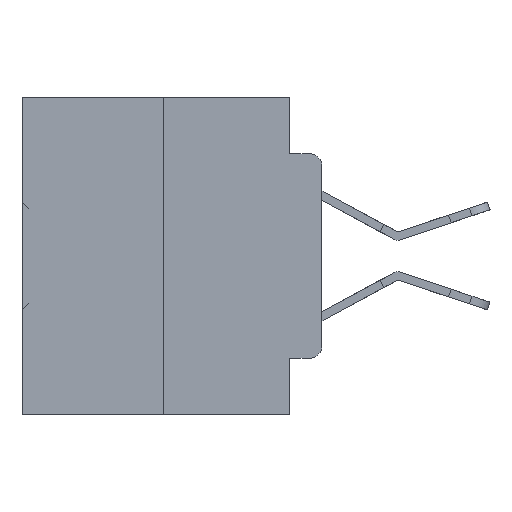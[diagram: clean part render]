
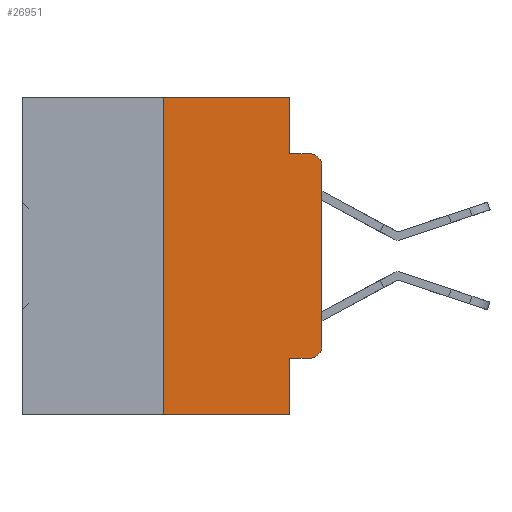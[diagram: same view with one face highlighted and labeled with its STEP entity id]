
A CAD part, left-side view. The second image highlights one B-rep face of the part: STEP entity #26951.
In plain terms, the highlighted planar face has unit normal (-1, 0, 0).
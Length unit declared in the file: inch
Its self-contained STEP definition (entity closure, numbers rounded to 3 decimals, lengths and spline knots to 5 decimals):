
#3 = EDGE_CURVE ( 'NONE', #21176, #24226, #10777, .T. ) ;
#64 = CARTESIAN_POINT ( 'NONE',  ( 0., 0.473, 0. ) ) ;
#279 = ORIENTED_EDGE ( 'NONE', *, *, #30904, .T. ) ;
#1422 = CARTESIAN_POINT ( 'NONE',  ( 0., 0.051, -0.0885 ) ) ;
#1730 = DIRECTION ( 'NONE',  ( 0., 0., 1. ) ) ;
#2903 = CIRCLE ( 'NONE', #6077, 0.02 ) ;
#4366 = CIRCLE ( 'NONE', #36384, 0.02 ) ;
#4468 = VECTOR ( 'NONE', #33080, 39.37008 ) ;
#5482 = LINE ( 'NONE', #11292, #4468 ) ;
#5577 = DIRECTION ( 'NONE',  ( 0., -1., 0. ) ) ;
#5899 = ORIENTED_EDGE ( 'NONE', *, *, #18908, .T. ) ;
#6077 = AXIS2_PLACEMENT_3D ( 'NONE', #33040, #14401, #36176 ) ;
#6322 = DIRECTION ( 'NONE',  ( -1., 0., 0. ) ) ;
#6934 = CARTESIAN_POINT ( 'NONE',  ( 0., 0.051, -0.4115 ) ) ;
#7149 = VECTOR ( 'NONE', #20381, 39.37008 ) ;
#7577 = CARTESIAN_POINT ( 'NONE',  ( 0., 0.051, 0. ) ) ;
#9055 = CARTESIAN_POINT ( 'NONE',  ( 0., 0., -0.3915 ) ) ;
#9959 = VECTOR ( 'NONE', #37285, 39.37008 ) ;
#10777 = LINE ( 'NONE', #7577, #18119 ) ;
#10796 = LINE ( 'NONE', #33046, #35670 ) ;
#10848 = CARTESIAN_POINT ( 'NONE',  ( 0., 0.051, -0.4115 ) ) ;
#11292 = CARTESIAN_POINT ( 'NONE',  ( 0., 0.473, -0.5 ) ) ;
#11466 = EDGE_CURVE ( 'NONE', #22764, #39345, #26602, .T. ) ;
#12318 = ORIENTED_EDGE ( 'NONE', *, *, #29073, .F. ) ;
#12628 = VERTEX_POINT ( 'NONE', #28226 ) ;
#14401 = DIRECTION ( 'NONE',  ( -1., 0., 0. ) ) ;
#15330 = VERTEX_POINT ( 'NONE', #18679 ) ;
#15375 = VECTOR ( 'NONE', #35049, 39.37008 ) ;
#15908 = VECTOR ( 'NONE', #5577, 39.37008 ) ;
#16170 = VERTEX_POINT ( 'NONE', #19553 ) ;
#16199 = AXIS2_PLACEMENT_3D ( 'NONE', #64, #37818, #19176 ) ;
#16276 = ORIENTED_EDGE ( 'NONE', *, *, #22108, .F. ) ;
#16366 = LINE ( 'NONE', #6934, #15375 ) ;
#16507 = LINE ( 'NONE', #1422, #7149 ) ;
#16768 = LINE ( 'NONE', #27586, #19677 ) ;
#17166 = CARTESIAN_POINT ( 'NONE',  ( 0., 0., -0.1085 ) ) ;
#17254 = CARTESIAN_POINT ( 'NONE',  ( 0., 0.25, 0. ) ) ;
#18119 = VECTOR ( 'NONE', #25619, 39.37008 ) ;
#18137 = CARTESIAN_POINT ( 'NONE',  ( 0., 0.473, 0. ) ) ;
#18679 = CARTESIAN_POINT ( 'NONE',  ( 0., 0.02, -0.0885 ) ) ;
#18908 = EDGE_CURVE ( 'NONE', #22764, #24226, #5482, .T. ) ;
#19041 = PLANE ( 'NONE',  #16199 ) ;
#19176 = DIRECTION ( 'NONE',  ( 0., 0., -1. ) ) ;
#19553 = CARTESIAN_POINT ( 'NONE',  ( 0., 0.051, 0. ) ) ;
#19677 = VECTOR ( 'NONE', #30671, 39.37008 ) ;
#20381 = DIRECTION ( 'NONE',  ( 0., -1., 0. ) ) ;
#20750 = EDGE_CURVE ( 'NONE', #39345, #16170, #24199, .T. ) ;
#21176 = VERTEX_POINT ( 'NONE', #10848 ) ;
#21931 = ORIENTED_EDGE ( 'NONE', *, *, #25823, .T. ) ;
#22108 = EDGE_CURVE ( 'NONE', #16170, #28282, #16768, .T. ) ;
#22236 = EDGE_CURVE ( 'NONE', #36190, #15330, #4366, .T. ) ;
#22699 = CARTESIAN_POINT ( 'NONE',  ( 0., 0.051, -0.5 ) ) ;
#22764 = VERTEX_POINT ( 'NONE', #37313 ) ;
#23187 = EDGE_CURVE ( 'NONE', #36437, #36190, #10796, .T. ) ;
#24199 = LINE ( 'NONE', #18137, #15908 ) ;
#24226 = VERTEX_POINT ( 'NONE', #22699 ) ;
#25109 = CARTESIAN_POINT ( 'NONE',  ( 0., 0.02, -0.1085 ) ) ;
#25619 = DIRECTION ( 'NONE',  ( 0., 0., -1. ) ) ;
#25823 = EDGE_CURVE ( 'NONE', #12628, #36437, #2903, .T. ) ;
#26602 = LINE ( 'NONE', #34161, #9959 ) ;
#26951 = ADVANCED_FACE ( 'NONE', ( #36657 ), #19041, .F. ) ;
#27586 = CARTESIAN_POINT ( 'NONE',  ( 0., 0.051, 0. ) ) ;
#28226 = CARTESIAN_POINT ( 'NONE',  ( 0., 0.02, -0.4115 ) ) ;
#28244 = DIRECTION ( 'NONE',  ( 0., 0., -1. ) ) ;
#28282 = VERTEX_POINT ( 'NONE', #29022 ) ;
#28566 = ORIENTED_EDGE ( 'NONE', *, *, #20750, .F. ) ;
#29022 = CARTESIAN_POINT ( 'NONE',  ( 0., 0.051, -0.0885 ) ) ;
#29073 = EDGE_CURVE ( 'NONE', #28282, #15330, #16507, .T. ) ;
#30671 = DIRECTION ( 'NONE',  ( 0., 0., -1. ) ) ;
#30904 = EDGE_CURVE ( 'NONE', #21176, #12628, #16366, .T. ) ;
#31549 = ORIENTED_EDGE ( 'NONE', *, *, #3, .F. ) ;
#33040 = CARTESIAN_POINT ( 'NONE',  ( 0., 0.02, -0.3915 ) ) ;
#33046 = CARTESIAN_POINT ( 'NONE',  ( 0., 0., 0. ) ) ;
#33080 = DIRECTION ( 'NONE',  ( 0., -1., 0. ) ) ;
#34161 = CARTESIAN_POINT ( 'NONE',  ( 0., 0.25, 0. ) ) ;
#34892 = ORIENTED_EDGE ( 'NONE', *, *, #22236, .T. ) ;
#35049 = DIRECTION ( 'NONE',  ( 0., -1., 0. ) ) ;
#35563 = ORIENTED_EDGE ( 'NONE', *, *, #11466, .F. ) ;
#35670 = VECTOR ( 'NONE', #1730, 39.37008 ) ;
#36176 = DIRECTION ( 'NONE',  ( 0., 0., -1. ) ) ;
#36190 = VERTEX_POINT ( 'NONE', #17166 ) ;
#36384 = AXIS2_PLACEMENT_3D ( 'NONE', #25109, #6322, #28244 ) ;
#36437 = VERTEX_POINT ( 'NONE', #9055 ) ;
#36657 = FACE_OUTER_BOUND ( 'NONE', #40009, .T. ) ;
#37285 = DIRECTION ( 'NONE',  ( 0., 0., 1. ) ) ;
#37313 = CARTESIAN_POINT ( 'NONE',  ( 0., 0.25, -0.5 ) ) ;
#37818 = DIRECTION ( 'NONE',  ( 1., 0., 0. ) ) ;
#38873 = ORIENTED_EDGE ( 'NONE', *, *, #23187, .T. ) ;
#39345 = VERTEX_POINT ( 'NONE', #17254 ) ;
#40009 = EDGE_LOOP ( 'NONE', ( #38873, #34892, #12318, #16276, #28566, #35563, #5899, #31549, #279, #21931 ) ) ;
